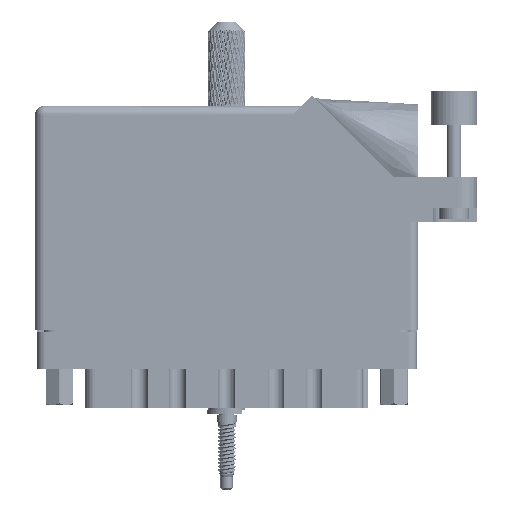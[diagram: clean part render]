
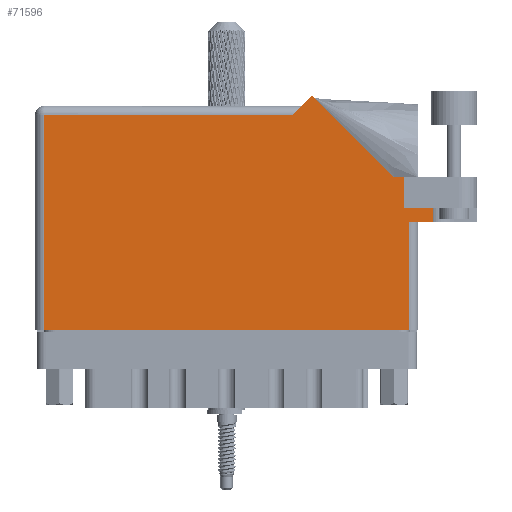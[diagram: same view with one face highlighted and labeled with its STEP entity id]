
A CAD part, front view. The second image highlights one B-rep face of the part: STEP entity #71596.
In plain terms, the highlighted face is planar.
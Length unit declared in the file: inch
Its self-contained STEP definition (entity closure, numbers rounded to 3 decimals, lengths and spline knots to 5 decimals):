
#118 = VECTOR ( 'NONE', #4908, 39.37008 ) ;
#758 = VECTOR ( 'NONE', #117177, 39.37008 ) ;
#2072 = EDGE_LOOP ( 'NONE', ( #55767, #82855, #63135, #109338, #110991, #102987, #12020, #58654, #123096, #100814, #29460 ) ) ;
#4012 = CARTESIAN_POINT ( 'NONE',  ( 2.512, 0.831, 0. ) ) ;
#4620 = VERTEX_POINT ( 'NONE', #68944 ) ;
#4908 = DIRECTION ( 'NONE',  ( 0., -1., 0. ) ) ;
#7595 = EDGE_CURVE ( 'NONE', #111496, #19194, #111809, .T. ) ;
#8606 = CARTESIAN_POINT ( 'NONE',  ( 1.757, 1.468, 0. ) ) ;
#11179 = LINE ( 'NONE', #67536, #25072 ) ;
#12020 = ORIENTED_EDGE ( 'NONE', *, *, #125416, .T. ) ;
#13119 = CARTESIAN_POINT ( 'NONE',  ( 1.88971, 1.60071, 0. ) ) ;
#15789 = VERTEX_POINT ( 'NONE', #41697 ) ;
#19194 = VERTEX_POINT ( 'NONE', #33371 ) ;
#24149 = EDGE_CURVE ( 'NONE', #33307, #111496, #76513, .T. ) ;
#24340 = DIRECTION ( 'NONE',  ( 0., 0., -1. ) ) ;
#25072 = VECTOR ( 'NONE', #27653, 39.37008 ) ;
#26864 = DIRECTION ( 'NONE',  ( 1., 0., 0. ) ) ;
#27653 = DIRECTION ( 'NONE',  ( 1., 0., 0. ) ) ;
#29460 = ORIENTED_EDGE ( 'NONE', *, *, #75927, .T. ) ;
#31757 = EDGE_CURVE ( 'NONE', #101750, #83383, #42660, .T. ) ;
#32054 = CARTESIAN_POINT ( 'NONE',  ( 0.062, 0., 0. ) ) ;
#33072 = EDGE_CURVE ( 'NONE', #33307, #15789, #115628, .T. ) ;
#33307 = VERTEX_POINT ( 'NONE', #87873 ) ;
#33371 = CARTESIAN_POINT ( 'NONE',  ( 2.7135, 0.737, 0. ) ) ;
#36685 = CARTESIAN_POINT ( 'NONE',  ( 2.55, 0.737, 0. ) ) ;
#39891 = VECTOR ( 'NONE', #50196, 39.37008 ) ;
#40749 = DIRECTION ( 'NONE',  ( 0., -1., 0. ) ) ;
#41697 = CARTESIAN_POINT ( 'NONE',  ( 2.512, 1.044, 0. ) ) ;
#42660 = LINE ( 'NONE', #92611, #59854 ) ;
#43806 = PLANE ( 'NONE',  #49968 ) ;
#47159 = VERTEX_POINT ( 'NONE', #36685 ) ;
#48457 = EDGE_CURVE ( 'NONE', #121355, #82036, #57979, .T. ) ;
#49968 = AXIS2_PLACEMENT_3D ( 'NONE', #95046, #24340, #104993 ) ;
#50196 = DIRECTION ( 'NONE',  ( 1., 0., 0. ) ) ;
#53266 = VECTOR ( 'NONE', #99385, 39.37008 ) ;
#55767 = ORIENTED_EDGE ( 'NONE', *, *, #69358, .T. ) ;
#57979 = LINE ( 'NONE', #115890, #758 ) ;
#58654 = ORIENTED_EDGE ( 'NONE', *, *, #48457, .T. ) ;
#59439 = CARTESIAN_POINT ( 'NONE',  ( 1.819, 1.53, 0. ) ) ;
#59854 = VECTOR ( 'NONE', #73078, 39.37008 ) ;
#60290 = CARTESIAN_POINT ( 'NONE',  ( 0.062, 0., 0. ) ) ;
#63135 = ORIENTED_EDGE ( 'NONE', *, *, #88590, .T. ) ;
#63160 = VECTOR ( 'NONE', #89358, 39.37008 ) ;
#67536 = CARTESIAN_POINT ( 'NONE',  ( 0., 0., 0. ) ) ;
#67797 = EDGE_CURVE ( 'NONE', #82036, #101750, #79706, .T. ) ;
#68759 = VECTOR ( 'NONE', #26864, 39.37008 ) ;
#68944 = CARTESIAN_POINT ( 'NONE',  ( 2.55, 0., 0. ) ) ;
#69358 = EDGE_CURVE ( 'NONE', #104251, #4620, #11179, .T. ) ;
#71596 = ADVANCED_FACE ( 'NONE', ( #113173 ), #43806, .F. ) ;
#73078 = DIRECTION ( 'NONE',  ( -1., 0., 0. ) ) ;
#75927 = EDGE_CURVE ( 'NONE', #83383, #104251, #102891, .T. ) ;
#76513 = LINE ( 'NONE', #96719, #68759 ) ;
#78883 = CARTESIAN_POINT ( 'NONE',  ( 2.612, 0.737, 0. ) ) ;
#79706 = LINE ( 'NONE', #59439, #53266 ) ;
#82036 = VERTEX_POINT ( 'NONE', #13119 ) ;
#82855 = ORIENTED_EDGE ( 'NONE', *, *, #97655, .T. ) ;
#83383 = VERTEX_POINT ( 'NONE', #128357 ) ;
#87873 = CARTESIAN_POINT ( 'NONE',  ( 2.512, 0.831, 0. ) ) ;
#88590 = EDGE_CURVE ( 'NONE', #47159, #19194, #97302, .T. ) ;
#89358 = DIRECTION ( 'NONE',  ( 0., 1., 0. ) ) ;
#89504 = CARTESIAN_POINT ( 'NONE',  ( 2.44642, 1.044, 0. ) ) ;
#92611 = CARTESIAN_POINT ( 'NONE',  ( 0., 1.468, 0. ) ) ;
#95046 = CARTESIAN_POINT ( 'NONE',  ( 0., 1.53, 0. ) ) ;
#96719 = CARTESIAN_POINT ( 'NONE',  ( 2.512, 0.831, 0. ) ) ;
#97302 = LINE ( 'NONE', #78883, #39891 ) ;
#97655 = EDGE_CURVE ( 'NONE', #4620, #47159, #105171, .T. ) ;
#99385 = DIRECTION ( 'NONE',  ( -0.707, -0.707, 0. ) ) ;
#100814 = ORIENTED_EDGE ( 'NONE', *, *, #31757, .T. ) ;
#101001 = VECTOR ( 'NONE', #127166, 39.37008 ) ;
#101750 = VERTEX_POINT ( 'NONE', #8606 ) ;
#102891 = LINE ( 'NONE', #32054, #121600 ) ;
#102987 = ORIENTED_EDGE ( 'NONE', *, *, #33072, .T. ) ;
#103728 = CARTESIAN_POINT ( 'NONE',  ( 2.7135, 1.16177, 0. ) ) ;
#104251 = VERTEX_POINT ( 'NONE', #60290 ) ;
#104993 = DIRECTION ( 'NONE',  ( -1., 0., 0. ) ) ;
#105171 = LINE ( 'NONE', #119304, #63160 ) ;
#107177 = LINE ( 'NONE', #128035, #101001 ) ;
#108460 = CARTESIAN_POINT ( 'NONE',  ( 2.7135, 0.831, 0. ) ) ;
#109338 = ORIENTED_EDGE ( 'NONE', *, *, #7595, .F. ) ;
#110991 = ORIENTED_EDGE ( 'NONE', *, *, #24149, .F. ) ;
#111496 = VERTEX_POINT ( 'NONE', #108460 ) ;
#111809 = LINE ( 'NONE', #103728, #118 ) ;
#113173 = FACE_OUTER_BOUND ( 'NONE', #2072, .T. ) ;
#115628 = LINE ( 'NONE', #4012, #123477 ) ;
#115890 = CARTESIAN_POINT ( 'NONE',  ( 2.44642, 1.044, 0. ) ) ;
#117177 = DIRECTION ( 'NONE',  ( -0.707, 0.707, 0. ) ) ;
#119304 = CARTESIAN_POINT ( 'NONE',  ( 2.55, 0.737, 0. ) ) ;
#121355 = VERTEX_POINT ( 'NONE', #89504 ) ;
#121600 = VECTOR ( 'NONE', #40749, 39.37008 ) ;
#121979 = DIRECTION ( 'NONE',  ( 0., 1., 0. ) ) ;
#123096 = ORIENTED_EDGE ( 'NONE', *, *, #67797, .T. ) ;
#123477 = VECTOR ( 'NONE', #121979, 39.37008 ) ;
#125416 = EDGE_CURVE ( 'NONE', #15789, #121355, #107177, .T. ) ;
#127166 = DIRECTION ( 'NONE',  ( -1., 0., 0. ) ) ;
#128035 = CARTESIAN_POINT ( 'NONE',  ( 3.012, 1.044, 0. ) ) ;
#128357 = CARTESIAN_POINT ( 'NONE',  ( 0.062, 1.468, 0. ) ) ;
